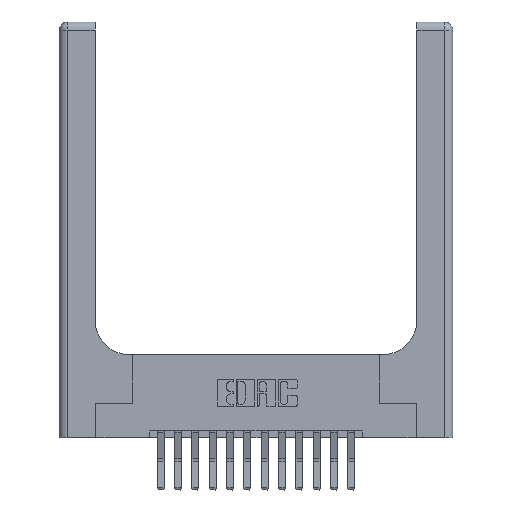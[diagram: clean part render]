
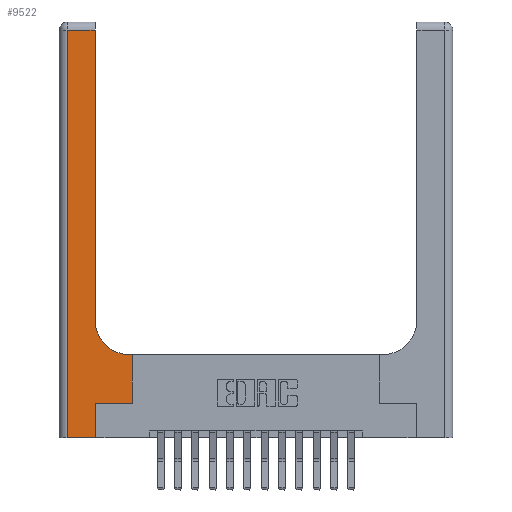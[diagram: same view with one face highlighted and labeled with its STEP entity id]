
A CAD part, top view. The second image highlights one B-rep face of the part: STEP entity #9522.
In plain terms, the highlighted planar face has unit normal (0, 0, 1).
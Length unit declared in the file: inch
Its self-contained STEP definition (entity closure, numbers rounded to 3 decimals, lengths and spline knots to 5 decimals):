
#222 = VECTOR ( 'NONE', #7090, 39.37008 ) ;
#679 = CARTESIAN_POINT ( 'NONE',  ( 0., 3., 0.37 ) ) ;
#909 = CARTESIAN_POINT ( 'NONE',  ( 0.26, 3., 0.37 ) ) ;
#1330 = DIRECTION ( 'NONE',  ( 1., 0., 0. ) ) ;
#1419 = EDGE_CURVE ( 'NONE', #9131, #10205, #17479, .T. ) ;
#2172 = CARTESIAN_POINT ( 'NONE',  ( 0.26, 2.94, 0.37 ) ) ;
#2317 = VERTEX_POINT ( 'NONE', #7270 ) ;
#2591 = EDGE_LOOP ( 'NONE', ( #2626, #10447, #16458, #13363, #13256, #15706, #12329, #7506, #11302 ) ) ;
#2626 = ORIENTED_EDGE ( 'NONE', *, *, #16765, .T. ) ;
#2640 = EDGE_CURVE ( 'NONE', #11000, #14894, #15447, .T. ) ;
#2743 = DIRECTION ( 'NONE',  ( -1., 0., 0. ) ) ;
#2893 = CARTESIAN_POINT ( 'NONE',  ( 0.51, 0.6, 0.37 ) ) ;
#3190 = VECTOR ( 'NONE', #2743, 39.37008 ) ;
#3247 = CARTESIAN_POINT ( 'NONE',  ( 0.26, 0.85, 0.37 ) ) ;
#3547 = CARTESIAN_POINT ( 'NONE',  ( 0.06, 0., 0.37 ) ) ;
#3572 = LINE ( 'NONE', #11781, #17066 ) ;
#3794 = LINE ( 'NONE', #12174, #3190 ) ;
#4003 = DIRECTION ( 'NONE',  ( 1., 0., 0. ) ) ;
#4532 = VERTEX_POINT ( 'NONE', #9195 ) ;
#4776 = DIRECTION ( 'NONE',  ( 0., 0., -1. ) ) ;
#4804 = LINE ( 'NONE', #7760, #11266 ) ;
#4872 = DIRECTION ( 'NONE',  ( -1., 0., 0. ) ) ;
#4974 = DIRECTION ( 'NONE',  ( -1., 0., 0. ) ) ;
#5520 = VERTEX_POINT ( 'NONE', #10455 ) ;
#6189 = EDGE_CURVE ( 'NONE', #5520, #4532, #4804, .T. ) ;
#6600 = VECTOR ( 'NONE', #17151, 39.37008 ) ;
#7090 = DIRECTION ( 'NONE',  ( 1., 0., 0. ) ) ;
#7270 = CARTESIAN_POINT ( 'NONE',  ( 0.06, 2.94, 0.37 ) ) ;
#7506 = ORIENTED_EDGE ( 'NONE', *, *, #11037, .T. ) ;
#7575 = CARTESIAN_POINT ( 'NONE',  ( 0.26, 0.6, 0.37 ) ) ;
#7755 = CARTESIAN_POINT ( 'NONE',  ( 0.265, 0., 0.37 ) ) ;
#7760 = CARTESIAN_POINT ( 'NONE',  ( 0.528, 0.25, 0.37 ) ) ;
#8274 = CARTESIAN_POINT ( 'NONE',  ( 0., 0., 0.37 ) ) ;
#9131 = VERTEX_POINT ( 'NONE', #2893 ) ;
#9195 = CARTESIAN_POINT ( 'NONE',  ( 0.528, 0.6, 0.37 ) ) ;
#9522 = ADVANCED_FACE ( 'NONE', ( #17018 ), #10221, .F. ) ;
#9618 = AXIS2_PLACEMENT_3D ( 'NONE', #679, #4776, #4872 ) ;
#10196 = EDGE_CURVE ( 'NONE', #14894, #5520, #13720, .T. ) ;
#10205 = VERTEX_POINT ( 'NONE', #3247 ) ;
#10221 = PLANE ( 'NONE',  #9618 ) ;
#10251 = DIRECTION ( 'NONE',  ( 0., 1., 0. ) ) ;
#10447 = ORIENTED_EDGE ( 'NONE', *, *, #15558, .T. ) ;
#10455 = CARTESIAN_POINT ( 'NONE',  ( 0.528, 0.25, 0.37 ) ) ;
#11000 = VERTEX_POINT ( 'NONE', #7755 ) ;
#11028 = VERTEX_POINT ( 'NONE', #3547 ) ;
#11037 = EDGE_CURVE ( 'NONE', #4532, #9131, #17130, .T. ) ;
#11266 = VECTOR ( 'NONE', #10251, 39.37008 ) ;
#11302 = ORIENTED_EDGE ( 'NONE', *, *, #1419, .T. ) ;
#11751 = EDGE_CURVE ( 'NONE', #11028, #11000, #16432, .T. ) ;
#11781 = CARTESIAN_POINT ( 'NONE',  ( 0.06, 3., 0.37 ) ) ;
#11903 = VECTOR ( 'NONE', #4974, 39.37008 ) ;
#12065 = CARTESIAN_POINT ( 'NONE',  ( 0.265, 0.25, 0.37 ) ) ;
#12174 = CARTESIAN_POINT ( 'NONE',  ( 0., 2.94, 0.37 ) ) ;
#12329 = ORIENTED_EDGE ( 'NONE', *, *, #6189, .T. ) ;
#12789 = DIRECTION ( 'NONE',  ( 0., 1., 0. ) ) ;
#13256 = ORIENTED_EDGE ( 'NONE', *, *, #2640, .T. ) ;
#13363 = ORIENTED_EDGE ( 'NONE', *, *, #11751, .T. ) ;
#13422 = LINE ( 'NONE', #909, #6600 ) ;
#13498 = AXIS2_PLACEMENT_3D ( 'NONE', #16090, #16171, #4003 ) ;
#13720 = LINE ( 'NONE', #15165, #222 ) ;
#13869 = VECTOR ( 'NONE', #1330, 39.37008 ) ;
#14894 = VERTEX_POINT ( 'NONE', #12065 ) ;
#15165 = CARTESIAN_POINT ( 'NONE',  ( 0.265, 0.25, 0.37 ) ) ;
#15412 = EDGE_CURVE ( 'NONE', #2317, #11028, #3572, .T. ) ;
#15447 = LINE ( 'NONE', #16695, #16745 ) ;
#15558 = EDGE_CURVE ( 'NONE', #16385, #2317, #3794, .T. ) ;
#15706 = ORIENTED_EDGE ( 'NONE', *, *, #10196, .T. ) ;
#16090 = CARTESIAN_POINT ( 'NONE',  ( 0.51, 0.85, 0.37 ) ) ;
#16171 = DIRECTION ( 'NONE',  ( 0., 0., -1. ) ) ;
#16385 = VERTEX_POINT ( 'NONE', #2172 ) ;
#16432 = LINE ( 'NONE', #8274, #13869 ) ;
#16458 = ORIENTED_EDGE ( 'NONE', *, *, #15412, .T. ) ;
#16695 = CARTESIAN_POINT ( 'NONE',  ( 0.265, 0., 0.37 ) ) ;
#16745 = VECTOR ( 'NONE', #12789, 39.37008 ) ;
#16765 = EDGE_CURVE ( 'NONE', #10205, #16385, #13422, .T. ) ;
#17018 = FACE_OUTER_BOUND ( 'NONE', #2591, .T. ) ;
#17066 = VECTOR ( 'NONE', #17152, 39.37008 ) ;
#17130 = LINE ( 'NONE', #7575, #11903 ) ;
#17151 = DIRECTION ( 'NONE',  ( 0., 1., 0. ) ) ;
#17152 = DIRECTION ( 'NONE',  ( 0., -1., 0. ) ) ;
#17479 = CIRCLE ( 'NONE', #13498, 0.25 ) ;
